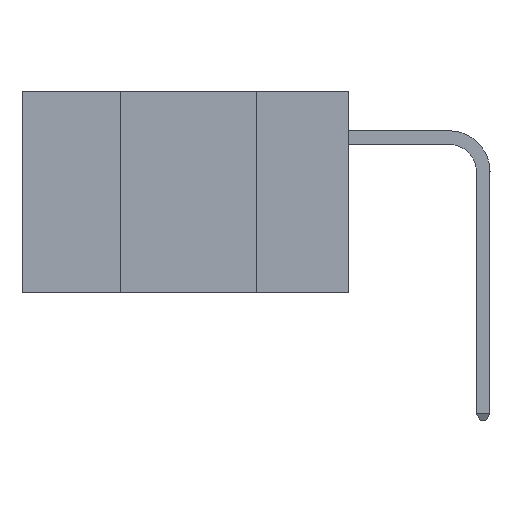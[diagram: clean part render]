
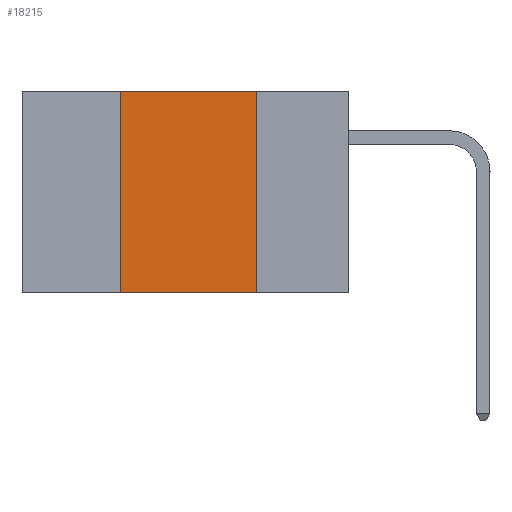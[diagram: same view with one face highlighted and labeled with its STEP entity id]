
A CAD part, left-side view. The second image highlights one B-rep face of the part: STEP entity #18215.
In plain terms, the highlighted planar face has unit normal (-1, 0, 0).
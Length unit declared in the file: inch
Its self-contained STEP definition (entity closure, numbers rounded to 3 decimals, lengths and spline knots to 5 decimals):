
#235 = EDGE_CURVE ( 'NONE', #32644, #16475, #22189, .T. ) ;
#1679 = CARTESIAN_POINT ( 'NONE',  ( 0., 0.6, 0. ) ) ;
#2113 = CARTESIAN_POINT ( 'NONE',  ( 0., 0.17, 0. ) ) ;
#3398 = DIRECTION ( 'NONE',  ( 0., -1., 0. ) ) ;
#3785 = CARTESIAN_POINT ( 'NONE',  ( 0., 0.42, 0. ) ) ;
#4246 = EDGE_LOOP ( 'NONE', ( #16820, #5387, #29052, #19876 ) ) ;
#5387 = ORIENTED_EDGE ( 'NONE', *, *, #11009, .F. ) ;
#6761 = DIRECTION ( 'NONE',  ( 0., -1., 0. ) ) ;
#7754 = CARTESIAN_POINT ( 'NONE',  ( 0., 0.6, 0. ) ) ;
#8150 = VERTEX_POINT ( 'NONE', #31941 ) ;
#8323 = CARTESIAN_POINT ( 'NONE',  ( 0., 0.6, -0.37 ) ) ;
#10925 = DIRECTION ( 'NONE',  ( 0., 0., -1. ) ) ;
#11009 = EDGE_CURVE ( 'NONE', #26831, #32644, #35155, .T. ) ;
#11741 = VECTOR ( 'NONE', #10925, 39.37008 ) ;
#12214 = VECTOR ( 'NONE', #3398, 39.37008 ) ;
#13185 = FACE_OUTER_BOUND ( 'NONE', #4246, .T. ) ;
#14875 = DIRECTION ( 'NONE',  ( 0., 0., 1. ) ) ;
#15380 = DIRECTION ( 'NONE',  ( 0., 0., -1. ) ) ;
#16475 = VERTEX_POINT ( 'NONE', #33117 ) ;
#16820 = ORIENTED_EDGE ( 'NONE', *, *, #235, .F. ) ;
#17276 = CARTESIAN_POINT ( 'NONE',  ( 0., 0.42, 0. ) ) ;
#17953 = LINE ( 'NONE', #3785, #35918 ) ;
#18215 = ADVANCED_FACE ( 'NONE', ( #13185 ), #35216, .F. ) ;
#19876 = ORIENTED_EDGE ( 'NONE', *, *, #32322, .T. ) ;
#22189 = LINE ( 'NONE', #35852, #11741 ) ;
#25221 = LINE ( 'NONE', #8323, #12214 ) ;
#26831 = VERTEX_POINT ( 'NONE', #17276 ) ;
#27191 = DIRECTION ( 'NONE',  ( 1., 0., 0. ) ) ;
#28508 = EDGE_CURVE ( 'NONE', #8150, #26831, #17953, .T. ) ;
#28555 = AXIS2_PLACEMENT_3D ( 'NONE', #7754, #27191, #15380 ) ;
#29052 = ORIENTED_EDGE ( 'NONE', *, *, #28508, .F. ) ;
#31941 = CARTESIAN_POINT ( 'NONE',  ( 0., 0.42, -0.37 ) ) ;
#32322 = EDGE_CURVE ( 'NONE', #8150, #16475, #25221, .T. ) ;
#32644 = VERTEX_POINT ( 'NONE', #2113 ) ;
#33117 = CARTESIAN_POINT ( 'NONE',  ( 0., 0.17, -0.37 ) ) ;
#35155 = LINE ( 'NONE', #1679, #35313 ) ;
#35216 = PLANE ( 'NONE',  #28555 ) ;
#35313 = VECTOR ( 'NONE', #6761, 39.37008 ) ;
#35852 = CARTESIAN_POINT ( 'NONE',  ( 0., 0.17, 0. ) ) ;
#35918 = VECTOR ( 'NONE', #14875, 39.37008 ) ;
